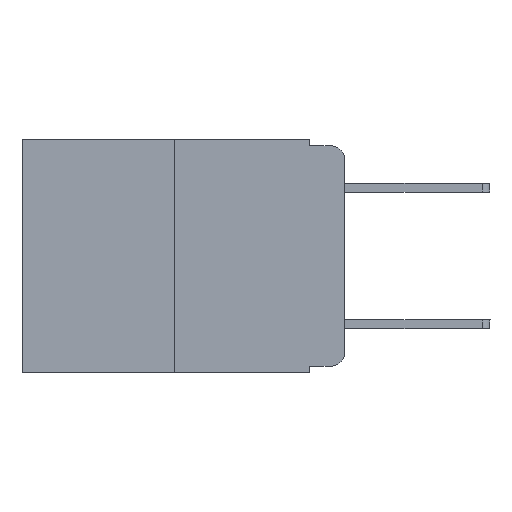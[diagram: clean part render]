
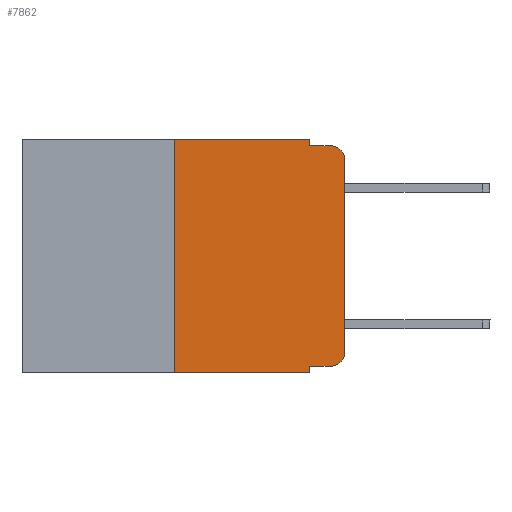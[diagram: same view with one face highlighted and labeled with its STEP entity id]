
A CAD part, left-side view. The second image highlights one B-rep face of the part: STEP entity #7862.
In plain terms, the highlighted planar face has unit normal (-1, 0, 0).
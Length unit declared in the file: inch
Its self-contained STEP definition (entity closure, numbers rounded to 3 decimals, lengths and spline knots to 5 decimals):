
#115 = PLANE ( 'NONE',  #12613 ) ;
#133 = DIRECTION ( 'NONE',  ( 0., -1., 0. ) ) ;
#266 = DIRECTION ( 'NONE',  ( 0., -1., 0. ) ) ;
#351 = AXIS2_PLACEMENT_3D ( 'NONE', #10297, #6654, #2975 ) ;
#679 = CARTESIAN_POINT ( 'NONE',  ( 0., 0.473, 0. ) ) ;
#1436 = EDGE_CURVE ( 'NONE', #8102, #9982, #11680, .T. ) ;
#1632 = EDGE_CURVE ( 'NONE', #4053, #13104, #5511, .T. ) ;
#2157 = CARTESIAN_POINT ( 'NONE',  ( 0., 0.051, 0. ) ) ;
#2328 = CARTESIAN_POINT ( 'NONE',  ( 0., 0., -0.03 ) ) ;
#2569 = CARTESIAN_POINT ( 'NONE',  ( 0., 0.051, 0. ) ) ;
#2787 = DIRECTION ( 'NONE',  ( 0., 0., 1. ) ) ;
#2804 = VECTOR ( 'NONE', #12008, 39.37008 ) ;
#2975 = DIRECTION ( 'NONE',  ( 0., 0., -1. ) ) ;
#3086 = CARTESIAN_POINT ( 'NONE',  ( 0., 0.051, -0.01 ) ) ;
#3334 = DIRECTION ( 'NONE',  ( 0., 0., -1. ) ) ;
#3720 = CARTESIAN_POINT ( 'NONE',  ( 0., 0.473, 0. ) ) ;
#4053 = VERTEX_POINT ( 'NONE', #12428 ) ;
#4191 = CARTESIAN_POINT ( 'NONE',  ( 0., 0.25, -0.343 ) ) ;
#4199 = VERTEX_POINT ( 'NONE', #4191 ) ;
#5322 = VECTOR ( 'NONE', #15125, 39.37008 ) ;
#5445 = ORIENTED_EDGE ( 'NONE', *, *, #1632, .F. ) ;
#5479 = CARTESIAN_POINT ( 'NONE',  ( 0., 0.051, -0.343 ) ) ;
#5511 = LINE ( 'NONE', #679, #10721 ) ;
#5576 = VERTEX_POINT ( 'NONE', #5479 ) ;
#5882 = EDGE_CURVE ( 'NONE', #4199, #4053, #11259, .T. ) ;
#5986 = LINE ( 'NONE', #7327, #2804 ) ;
#5988 = EDGE_CURVE ( 'NONE', #7262, #11716, #13716, .T. ) ;
#6160 = VECTOR ( 'NONE', #10950, 39.37008 ) ;
#6339 = ORIENTED_EDGE ( 'NONE', *, *, #6590, .T. ) ;
#6341 = EDGE_CURVE ( 'NONE', #7262, #5576, #13696, .T. ) ;
#6498 = EDGE_CURVE ( 'NONE', #11716, #14192, #14798, .T. ) ;
#6545 = ORIENTED_EDGE ( 'NONE', *, *, #5882, .F. ) ;
#6590 = EDGE_CURVE ( 'NONE', #14192, #8396, #5986, .T. ) ;
#6654 = DIRECTION ( 'NONE',  ( -1., 0., 0. ) ) ;
#7206 = EDGE_CURVE ( 'NONE', #13104, #8102, #11961, .T. ) ;
#7262 = VERTEX_POINT ( 'NONE', #14734 ) ;
#7327 = CARTESIAN_POINT ( 'NONE',  ( 0., 0., 0. ) ) ;
#7332 = VECTOR ( 'NONE', #14963, 39.37008 ) ;
#7431 = VECTOR ( 'NONE', #133, 39.37008 ) ;
#7723 = CARTESIAN_POINT ( 'NONE',  ( 0., 0.25, 0. ) ) ;
#7786 = ORIENTED_EDGE ( 'NONE', *, *, #7206, .F. ) ;
#7862 = ADVANCED_FACE ( 'NONE', ( #13259 ), #115, .F. ) ;
#8102 = VERTEX_POINT ( 'NONE', #3086 ) ;
#8396 = VERTEX_POINT ( 'NONE', #2328 ) ;
#8527 = DIRECTION ( 'NONE',  ( 0., 0., -1. ) ) ;
#9419 = ORIENTED_EDGE ( 'NONE', *, *, #11570, .T. ) ;
#9502 = AXIS2_PLACEMENT_3D ( 'NONE', #10496, #11610, #3334 ) ;
#9982 = VERTEX_POINT ( 'NONE', #14697 ) ;
#10047 = CARTESIAN_POINT ( 'NONE',  ( 0., 0., -0.313 ) ) ;
#10297 = CARTESIAN_POINT ( 'NONE',  ( 0., 0.02, -0.03 ) ) ;
#10445 = ORIENTED_EDGE ( 'NONE', *, *, #11976, .T. ) ;
#10496 = CARTESIAN_POINT ( 'NONE',  ( 0., 0.02, -0.313 ) ) ;
#10501 = VECTOR ( 'NONE', #266, 39.37008 ) ;
#10721 = VECTOR ( 'NONE', #15218, 39.37008 ) ;
#10950 = DIRECTION ( 'NONE',  ( 0., 0., -1. ) ) ;
#11259 = LINE ( 'NONE', #7723, #12954 ) ;
#11411 = CARTESIAN_POINT ( 'NONE',  ( 0., 0.051, 0. ) ) ;
#11566 = CARTESIAN_POINT ( 'NONE',  ( 0., 0.051, -0.01 ) ) ;
#11570 = EDGE_CURVE ( 'NONE', #8396, #9982, #12672, .T. ) ;
#11610 = DIRECTION ( 'NONE',  ( -1., 0., 0. ) ) ;
#11680 = LINE ( 'NONE', #11566, #5322 ) ;
#11702 = CARTESIAN_POINT ( 'NONE',  ( 0., 0.02, -0.333 ) ) ;
#11716 = VERTEX_POINT ( 'NONE', #11702 ) ;
#11961 = LINE ( 'NONE', #2569, #6160 ) ;
#11976 = EDGE_CURVE ( 'NONE', #4199, #5576, #13030, .T. ) ;
#12008 = DIRECTION ( 'NONE',  ( 0., 0., 1. ) ) ;
#12105 = CARTESIAN_POINT ( 'NONE',  ( 0., 0.473, -0.343 ) ) ;
#12428 = CARTESIAN_POINT ( 'NONE',  ( 0., 0.25, 0. ) ) ;
#12613 = AXIS2_PLACEMENT_3D ( 'NONE', #3720, #13349, #8527 ) ;
#12642 = EDGE_LOOP ( 'NONE', ( #6339, #9419, #14589, #7786, #5445, #6545, #10445, #12938, #14817, #13034 ) ) ;
#12672 = CIRCLE ( 'NONE', #351, 0.02 ) ;
#12938 = ORIENTED_EDGE ( 'NONE', *, *, #6341, .F. ) ;
#12954 = VECTOR ( 'NONE', #2787, 39.37008 ) ;
#13030 = LINE ( 'NONE', #12105, #7431 ) ;
#13034 = ORIENTED_EDGE ( 'NONE', *, *, #6498, .T. ) ;
#13104 = VERTEX_POINT ( 'NONE', #2157 ) ;
#13259 = FACE_OUTER_BOUND ( 'NONE', #12642, .T. ) ;
#13349 = DIRECTION ( 'NONE',  ( 1., 0., 0. ) ) ;
#13696 = LINE ( 'NONE', #11411, #7332 ) ;
#13716 = LINE ( 'NONE', #14923, #10501 ) ;
#14192 = VERTEX_POINT ( 'NONE', #10047 ) ;
#14589 = ORIENTED_EDGE ( 'NONE', *, *, #1436, .F. ) ;
#14697 = CARTESIAN_POINT ( 'NONE',  ( 0., 0.02, -0.01 ) ) ;
#14734 = CARTESIAN_POINT ( 'NONE',  ( 0., 0.051, -0.333 ) ) ;
#14798 = CIRCLE ( 'NONE', #9502, 0.02 ) ;
#14817 = ORIENTED_EDGE ( 'NONE', *, *, #5988, .T. ) ;
#14923 = CARTESIAN_POINT ( 'NONE',  ( 0., 0.051, -0.333 ) ) ;
#14963 = DIRECTION ( 'NONE',  ( 0., 0., -1. ) ) ;
#15125 = DIRECTION ( 'NONE',  ( 0., -1., 0. ) ) ;
#15218 = DIRECTION ( 'NONE',  ( 0., -1., 0. ) ) ;
